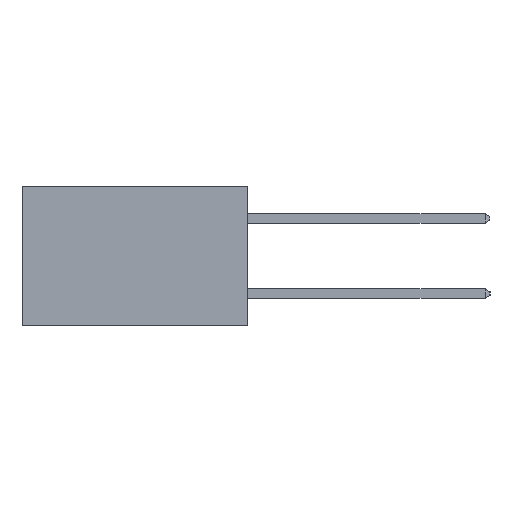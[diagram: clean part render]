
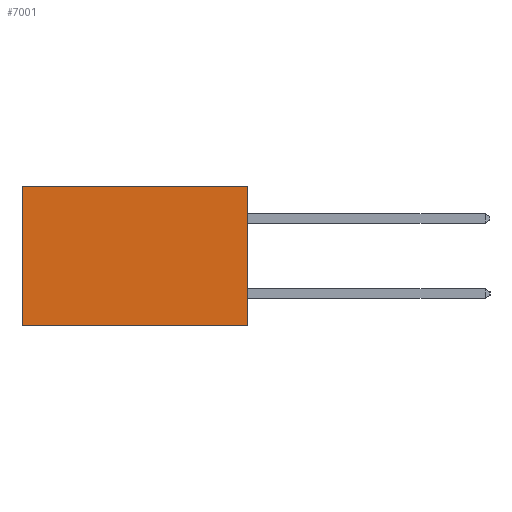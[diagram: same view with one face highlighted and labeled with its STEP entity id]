
A CAD part, left-side view. The second image highlights one B-rep face of the part: STEP entity #7001.
In plain terms, the highlighted planar face has unit normal (-1, 0, 0).
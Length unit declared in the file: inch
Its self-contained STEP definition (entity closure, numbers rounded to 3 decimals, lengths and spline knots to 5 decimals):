
#662 = VERTEX_POINT ( 'NONE', #18473 ) ;
#1420 = CARTESIAN_POINT ( 'NONE',  ( 0.2615, 0., -0.37 ) ) ;
#1560 = CARTESIAN_POINT ( 'NONE',  ( 0.2615, 0., 0. ) ) ;
#2013 = ORIENTED_EDGE ( 'NONE', *, *, #17795, .T. ) ;
#2033 = VECTOR ( 'NONE', #10351, 39.37008 ) ;
#2520 = VERTEX_POINT ( 'NONE', #6565 ) ;
#2671 = CARTESIAN_POINT ( 'NONE',  ( 0.2615, 0.6, -0.37 ) ) ;
#2853 = EDGE_CURVE ( 'NONE', #2520, #8031, #13960, .T. ) ;
#3287 = DIRECTION ( 'NONE',  ( 0., 0., -1. ) ) ;
#3374 = AXIS2_PLACEMENT_3D ( 'NONE', #17385, #8989, #6170 ) ;
#4226 = DIRECTION ( 'NONE',  ( 0., 0., -1. ) ) ;
#4625 = CARTESIAN_POINT ( 'NONE',  ( 0.2615, 0.6, -0.37 ) ) ;
#5830 = PLANE ( 'NONE',  #3374 ) ;
#5944 = LINE ( 'NONE', #1560, #2033 ) ;
#6170 = DIRECTION ( 'NONE',  ( 0., 0., -1. ) ) ;
#6565 = CARTESIAN_POINT ( 'NONE',  ( 0.2615, 0.6, 0. ) ) ;
#6883 = VECTOR ( 'NONE', #4226, 39.37008 ) ;
#7001 = ADVANCED_FACE ( 'NONE', ( #12654 ), #5830, .F. ) ;
#7866 = VECTOR ( 'NONE', #3287, 39.37008 ) ;
#8031 = VERTEX_POINT ( 'NONE', #2671 ) ;
#8122 = ORIENTED_EDGE ( 'NONE', *, *, #2853, .T. ) ;
#8475 = EDGE_LOOP ( 'NONE', ( #8122, #9962, #14005, #2013 ) ) ;
#8989 = DIRECTION ( 'NONE',  ( 1., 0., 0. ) ) ;
#9337 = EDGE_CURVE ( 'NONE', #10530, #8031, #12138, .T. ) ;
#9962 = ORIENTED_EDGE ( 'NONE', *, *, #9337, .F. ) ;
#10351 = DIRECTION ( 'NONE',  ( 0., 1., 0. ) ) ;
#10516 = CARTESIAN_POINT ( 'NONE',  ( 0.2615, 0., -0.37 ) ) ;
#10530 = VERTEX_POINT ( 'NONE', #1420 ) ;
#11089 = DIRECTION ( 'NONE',  ( 0., 1., 0. ) ) ;
#11317 = EDGE_CURVE ( 'NONE', #662, #10530, #15378, .T. ) ;
#11696 = VECTOR ( 'NONE', #11089, 39.37008 ) ;
#12138 = LINE ( 'NONE', #12496, #11696 ) ;
#12496 = CARTESIAN_POINT ( 'NONE',  ( 0.2615, 0., -0.37 ) ) ;
#12654 = FACE_OUTER_BOUND ( 'NONE', #8475, .T. ) ;
#13960 = LINE ( 'NONE', #4625, #6883 ) ;
#14005 = ORIENTED_EDGE ( 'NONE', *, *, #11317, .F. ) ;
#15378 = LINE ( 'NONE', #10516, #7866 ) ;
#17385 = CARTESIAN_POINT ( 'NONE',  ( 0.2615, 0., -0.37 ) ) ;
#17795 = EDGE_CURVE ( 'NONE', #662, #2520, #5944, .T. ) ;
#18473 = CARTESIAN_POINT ( 'NONE',  ( 0.2615, 0., 0. ) ) ;
